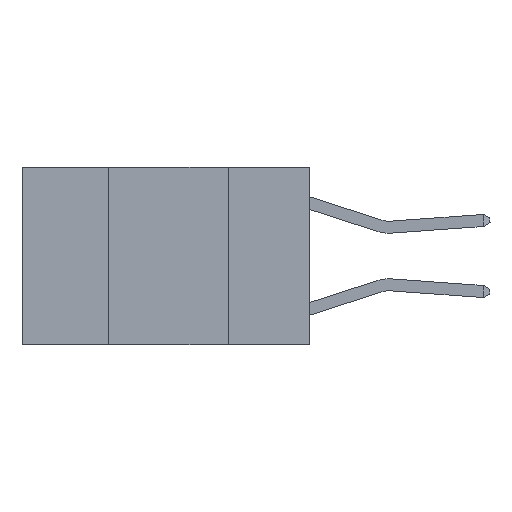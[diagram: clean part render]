
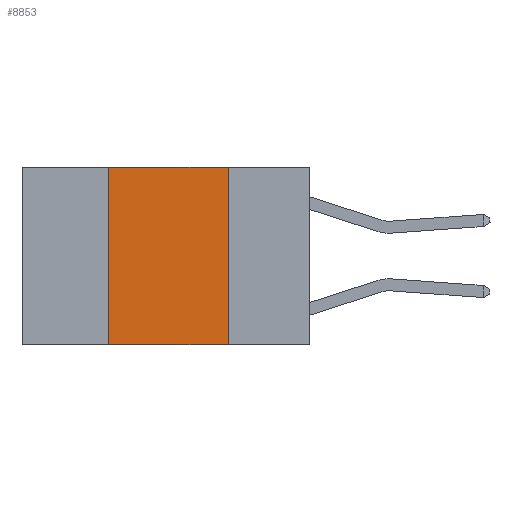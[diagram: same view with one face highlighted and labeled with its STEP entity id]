
A CAD part, left-side view. The second image highlights one B-rep face of the part: STEP entity #8853.
In plain terms, the highlighted planar face has unit normal (-1, 0, 0).
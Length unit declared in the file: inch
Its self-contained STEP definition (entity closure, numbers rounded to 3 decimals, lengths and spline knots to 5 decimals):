
#135 = LINE ( 'NONE', #18891, #11517 ) ;
#374 = CARTESIAN_POINT ( 'NONE',  ( 0., 0.42, -0.37 ) ) ;
#464 = DIRECTION ( 'NONE',  ( 0., 0., -1. ) ) ;
#489 = EDGE_CURVE ( 'NONE', #2450, #5916, #135, .T. ) ;
#940 = CARTESIAN_POINT ( 'NONE',  ( 0., 0.6, 0. ) ) ;
#1679 = DIRECTION ( 'NONE',  ( 0., 0., 1. ) ) ;
#1771 = ORIENTED_EDGE ( 'NONE', *, *, #14343, .F. ) ;
#2081 = VERTEX_POINT ( 'NONE', #15833 ) ;
#2450 = VERTEX_POINT ( 'NONE', #374 ) ;
#2587 = FACE_OUTER_BOUND ( 'NONE', #8877, .T. ) ;
#3232 = CARTESIAN_POINT ( 'NONE',  ( 0., 0.6, 0. ) ) ;
#4755 = PLANE ( 'NONE',  #17485 ) ;
#5509 = LINE ( 'NONE', #15165, #14237 ) ;
#5560 = VERTEX_POINT ( 'NONE', #11428 ) ;
#5670 = DIRECTION ( 'NONE',  ( 0., -1., 0. ) ) ;
#5916 = VERTEX_POINT ( 'NONE', #15067 ) ;
#6135 = ORIENTED_EDGE ( 'NONE', *, *, #9502, .F. ) ;
#7780 = DIRECTION ( 'NONE',  ( 0., 0., -1. ) ) ;
#8853 = ADVANCED_FACE ( 'NONE', ( #2587 ), #4755, .F. ) ;
#8877 = EDGE_LOOP ( 'NONE', ( #1771, #13921, #6135, #10854 ) ) ;
#9177 = CARTESIAN_POINT ( 'NONE',  ( 0., 0.42, 0. ) ) ;
#9502 = EDGE_CURVE ( 'NONE', #2450, #2081, #14578, .T. ) ;
#10739 = VECTOR ( 'NONE', #1679, 39.37008 ) ;
#10854 = ORIENTED_EDGE ( 'NONE', *, *, #489, .T. ) ;
#11428 = CARTESIAN_POINT ( 'NONE',  ( 0., 0.17, 0. ) ) ;
#11517 = VECTOR ( 'NONE', #5670, 39.37008 ) ;
#11594 = VECTOR ( 'NONE', #14263, 39.37008 ) ;
#12052 = LINE ( 'NONE', #940, #11594 ) ;
#12735 = EDGE_CURVE ( 'NONE', #2081, #5560, #12052, .T. ) ;
#13921 = ORIENTED_EDGE ( 'NONE', *, *, #12735, .F. ) ;
#14237 = VECTOR ( 'NONE', #464, 39.37008 ) ;
#14263 = DIRECTION ( 'NONE',  ( 0., -1., 0. ) ) ;
#14343 = EDGE_CURVE ( 'NONE', #5560, #5916, #5509, .T. ) ;
#14578 = LINE ( 'NONE', #9177, #10739 ) ;
#15067 = CARTESIAN_POINT ( 'NONE',  ( 0., 0.17, -0.37 ) ) ;
#15165 = CARTESIAN_POINT ( 'NONE',  ( 0., 0.17, 0. ) ) ;
#15833 = CARTESIAN_POINT ( 'NONE',  ( 0., 0.42, 0. ) ) ;
#16461 = DIRECTION ( 'NONE',  ( 1., 0., 0. ) ) ;
#17485 = AXIS2_PLACEMENT_3D ( 'NONE', #3232, #16461, #7780 ) ;
#18891 = CARTESIAN_POINT ( 'NONE',  ( 0., 0.6, -0.37 ) ) ;
